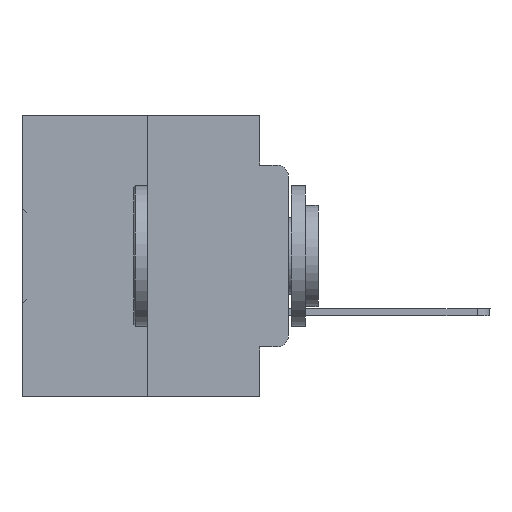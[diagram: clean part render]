
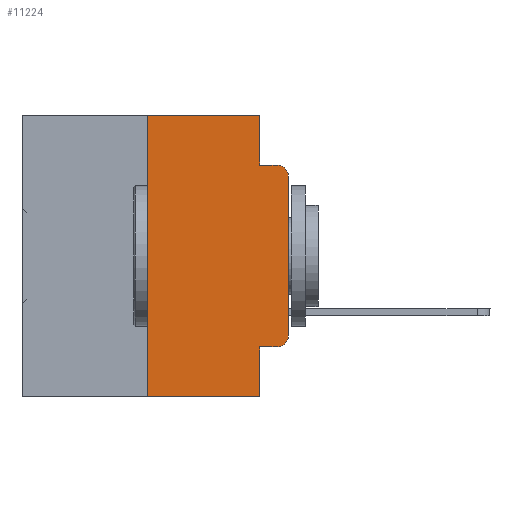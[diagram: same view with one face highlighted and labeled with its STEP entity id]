
A CAD part, left-side view. The second image highlights one B-rep face of the part: STEP entity #11224.
In plain terms, the highlighted planar face has unit normal (-1, 0, 0).
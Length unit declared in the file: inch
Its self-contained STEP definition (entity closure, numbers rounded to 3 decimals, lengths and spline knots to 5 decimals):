
#626 = VECTOR ( 'NONE', #12818, 39.37008 ) ;
#1283 = CARTESIAN_POINT ( 'NONE',  ( 0., 0., -0.1085 ) ) ;
#1952 = CARTESIAN_POINT ( 'NONE',  ( 0., 0.051, -0.4115 ) ) ;
#2150 = EDGE_CURVE ( 'NONE', #16758, #16878, #4331, .T. ) ;
#2917 = ORIENTED_EDGE ( 'NONE', *, *, #11763, .F. ) ;
#3540 = CARTESIAN_POINT ( 'NONE',  ( 0., 0.02, -0.1085 ) ) ;
#4184 = VECTOR ( 'NONE', #10209, 39.37008 ) ;
#4331 = CIRCLE ( 'NONE', #7686, 0.02 ) ;
#4465 = AXIS2_PLACEMENT_3D ( 'NONE', #13540, #23762, #34524 ) ;
#4484 = VECTOR ( 'NONE', #11044, 39.37008 ) ;
#4525 = LINE ( 'NONE', #17571, #626 ) ;
#4814 = CIRCLE ( 'NONE', #10462, 0.02 ) ;
#4857 = LINE ( 'NONE', #32472, #27310 ) ;
#6583 = VERTEX_POINT ( 'NONE', #19601 ) ;
#6625 = LINE ( 'NONE', #17392, #8841 ) ;
#6642 = EDGE_CURVE ( 'NONE', #30467, #19734, #17971, .T. ) ;
#7200 = CARTESIAN_POINT ( 'NONE',  ( 0., 0.473, 0. ) ) ;
#7321 = EDGE_CURVE ( 'NONE', #10446, #16758, #12233, .T. ) ;
#7686 = AXIS2_PLACEMENT_3D ( 'NONE', #3540, #30156, #8462 ) ;
#8376 = LINE ( 'NONE', #24955, #15937 ) ;
#8462 = DIRECTION ( 'NONE',  ( 0., 0., -1. ) ) ;
#8687 = EDGE_CURVE ( 'NONE', #24474, #12570, #6625, .T. ) ;
#8841 = VECTOR ( 'NONE', #28134, 39.37008 ) ;
#9310 = DIRECTION ( 'NONE',  ( -1., 0., 0. ) ) ;
#9918 = VECTOR ( 'NONE', #28549, 39.37008 ) ;
#10209 = DIRECTION ( 'NONE',  ( 0., -1., 0. ) ) ;
#10446 = VERTEX_POINT ( 'NONE', #29841 ) ;
#10462 = AXIS2_PLACEMENT_3D ( 'NONE', #20411, #9310, #17256 ) ;
#11044 = DIRECTION ( 'NONE',  ( 0., -1., 0. ) ) ;
#11224 = ADVANCED_FACE ( 'NONE', ( #13200 ), #13025, .F. ) ;
#11256 = ORIENTED_EDGE ( 'NONE', *, *, #6642, .T. ) ;
#11763 = EDGE_CURVE ( 'NONE', #12570, #16878, #24945, .T. ) ;
#11864 = CARTESIAN_POINT ( 'NONE',  ( 0., 0.02, -0.4115 ) ) ;
#12233 = LINE ( 'NONE', #15040, #32952 ) ;
#12570 = VERTEX_POINT ( 'NONE', #29410 ) ;
#12818 = DIRECTION ( 'NONE',  ( 0., -1., 0. ) ) ;
#13025 = PLANE ( 'NONE',  #4465 ) ;
#13200 = FACE_OUTER_BOUND ( 'NONE', #28415, .T. ) ;
#13540 = CARTESIAN_POINT ( 'NONE',  ( 0., 0.473, 0. ) ) ;
#14113 = EDGE_CURVE ( 'NONE', #25875, #6583, #4525, .T. ) ;
#15040 = CARTESIAN_POINT ( 'NONE',  ( 0., 0., 0. ) ) ;
#15937 = VECTOR ( 'NONE', #33062, 39.37008 ) ;
#16377 = ORIENTED_EDGE ( 'NONE', *, *, #2150, .T. ) ;
#16407 = CARTESIAN_POINT ( 'NONE',  ( 0., 0.25, 0. ) ) ;
#16758 = VERTEX_POINT ( 'NONE', #1283 ) ;
#16878 = VERTEX_POINT ( 'NONE', #31567 ) ;
#17256 = DIRECTION ( 'NONE',  ( 0., 0., -1. ) ) ;
#17392 = CARTESIAN_POINT ( 'NONE',  ( 0., 0.051, 0. ) ) ;
#17571 = CARTESIAN_POINT ( 'NONE',  ( 0., 0.473, -0.5 ) ) ;
#17971 = LINE ( 'NONE', #1952, #9918 ) ;
#19091 = DIRECTION ( 'NONE',  ( 0., 0., 1. ) ) ;
#19480 = ORIENTED_EDGE ( 'NONE', *, *, #21534, .F. ) ;
#19601 = CARTESIAN_POINT ( 'NONE',  ( 0., 0.051, -0.5 ) ) ;
#19688 = ORIENTED_EDGE ( 'NONE', *, *, #23813, .F. ) ;
#19734 = VERTEX_POINT ( 'NONE', #11864 ) ;
#19911 = VERTEX_POINT ( 'NONE', #16407 ) ;
#20378 = EDGE_CURVE ( 'NONE', #30467, #6583, #8376, .T. ) ;
#20411 = CARTESIAN_POINT ( 'NONE',  ( 0., 0.02, -0.3915 ) ) ;
#21534 = EDGE_CURVE ( 'NONE', #19911, #24474, #26429, .T. ) ;
#22533 = ORIENTED_EDGE ( 'NONE', *, *, #8687, .F. ) ;
#23044 = ORIENTED_EDGE ( 'NONE', *, *, #14113, .T. ) ;
#23248 = EDGE_CURVE ( 'NONE', #19734, #10446, #4814, .T. ) ;
#23762 = DIRECTION ( 'NONE',  ( 1., 0., 0. ) ) ;
#23813 = EDGE_CURVE ( 'NONE', #25875, #19911, #4857, .T. ) ;
#24195 = ORIENTED_EDGE ( 'NONE', *, *, #7321, .T. ) ;
#24474 = VERTEX_POINT ( 'NONE', #28860 ) ;
#24945 = LINE ( 'NONE', #27242, #4484 ) ;
#24955 = CARTESIAN_POINT ( 'NONE',  ( 0., 0.051, 0. ) ) ;
#25495 = ORIENTED_EDGE ( 'NONE', *, *, #20378, .F. ) ;
#25621 = DIRECTION ( 'NONE',  ( 0., 0., 1. ) ) ;
#25875 = VERTEX_POINT ( 'NONE', #34521 ) ;
#26429 = LINE ( 'NONE', #7200, #4184 ) ;
#27242 = CARTESIAN_POINT ( 'NONE',  ( 0., 0.051, -0.0885 ) ) ;
#27310 = VECTOR ( 'NONE', #19091, 39.37008 ) ;
#27713 = ORIENTED_EDGE ( 'NONE', *, *, #23248, .T. ) ;
#28134 = DIRECTION ( 'NONE',  ( 0., 0., -1. ) ) ;
#28415 = EDGE_LOOP ( 'NONE', ( #24195, #16377, #2917, #22533, #19480, #19688, #23044, #25495, #11256, #27713 ) ) ;
#28549 = DIRECTION ( 'NONE',  ( 0., -1., 0. ) ) ;
#28860 = CARTESIAN_POINT ( 'NONE',  ( 0., 0.051, 0. ) ) ;
#29410 = CARTESIAN_POINT ( 'NONE',  ( 0., 0.051, -0.0885 ) ) ;
#29841 = CARTESIAN_POINT ( 'NONE',  ( 0., 0., -0.3915 ) ) ;
#30156 = DIRECTION ( 'NONE',  ( -1., 0., 0. ) ) ;
#30467 = VERTEX_POINT ( 'NONE', #33017 ) ;
#31567 = CARTESIAN_POINT ( 'NONE',  ( 0., 0.02, -0.0885 ) ) ;
#32472 = CARTESIAN_POINT ( 'NONE',  ( 0., 0.25, 0. ) ) ;
#32952 = VECTOR ( 'NONE', #25621, 39.37008 ) ;
#33017 = CARTESIAN_POINT ( 'NONE',  ( 0., 0.051, -0.4115 ) ) ;
#33062 = DIRECTION ( 'NONE',  ( 0., 0., -1. ) ) ;
#34521 = CARTESIAN_POINT ( 'NONE',  ( 0., 0.25, -0.5 ) ) ;
#34524 = DIRECTION ( 'NONE',  ( 0., 0., -1. ) ) ;
